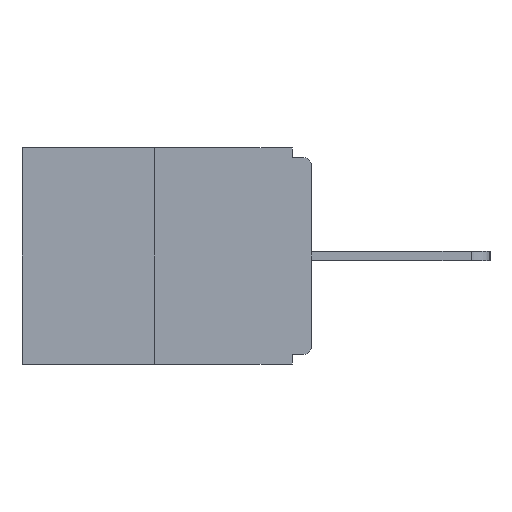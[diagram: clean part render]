
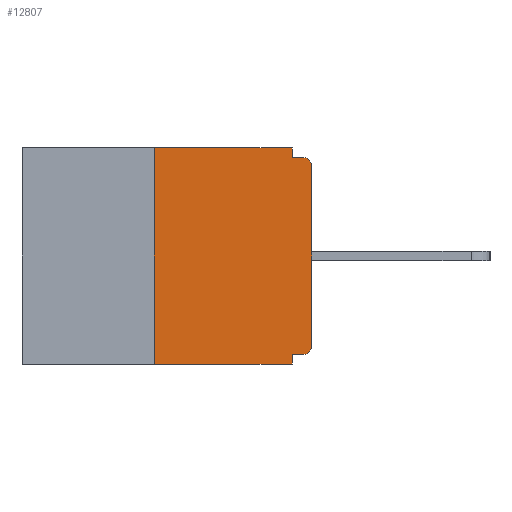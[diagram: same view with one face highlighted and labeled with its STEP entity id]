
A CAD part, left-side view. The second image highlights one B-rep face of the part: STEP entity #12807.
In plain terms, the highlighted planar face has unit normal (-1, 0, 0).
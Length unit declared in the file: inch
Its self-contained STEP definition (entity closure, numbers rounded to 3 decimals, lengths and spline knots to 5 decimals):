
#68 = CARTESIAN_POINT ( 'NONE',  ( 0., 0.031, 0. ) ) ;
#231 = AXIS2_PLACEMENT_3D ( 'NONE', #5222, #12648, #6312 ) ;
#589 = VERTEX_POINT ( 'NONE', #12794 ) ;
#752 = VECTOR ( 'NONE', #6473, 39.37008 ) ;
#1267 = VERTEX_POINT ( 'NONE', #9443 ) ;
#1361 = EDGE_CURVE ( 'NONE', #7565, #2502, #13836, .T. ) ;
#1569 = CARTESIAN_POINT ( 'NONE',  ( 0., 0., -0.313 ) ) ;
#1834 = ORIENTED_EDGE ( 'NONE', *, *, #4089, .F. ) ;
#2036 = VERTEX_POINT ( 'NONE', #1569 ) ;
#2199 = ORIENTED_EDGE ( 'NONE', *, *, #1361, .T. ) ;
#2500 = CARTESIAN_POINT ( 'NONE',  ( 0., 0.015, -0.015 ) ) ;
#2502 = VERTEX_POINT ( 'NONE', #7137 ) ;
#2579 = CARTESIAN_POINT ( 'NONE',  ( 0., 0., -0.03 ) ) ;
#2752 = CARTESIAN_POINT ( 'NONE',  ( 0., 0.46, 0. ) ) ;
#2889 = DIRECTION ( 'NONE',  ( 0., 0., -1. ) ) ;
#2912 = DIRECTION ( 'NONE',  ( 0., -1., 0. ) ) ;
#3065 = EDGE_LOOP ( 'NONE', ( #12920, #1834, #2199, #13422, #8104, #5618, #12589, #13583, #11748, #3576 ) ) ;
#3076 = CARTESIAN_POINT ( 'NONE',  ( 0., 0.46, -0.343 ) ) ;
#3139 = VECTOR ( 'NONE', #6002, 39.37008 ) ;
#3576 = ORIENTED_EDGE ( 'NONE', *, *, #10837, .F. ) ;
#3677 = CARTESIAN_POINT ( 'NONE',  ( 0., 0.015, -0.03 ) ) ;
#3810 = CARTESIAN_POINT ( 'NONE',  ( 0., 0.46, 0. ) ) ;
#3862 = DIRECTION ( 'NONE',  ( 0., 0., -1. ) ) ;
#4089 = EDGE_CURVE ( 'NONE', #7565, #5576, #6040, .T. ) ;
#4292 = CARTESIAN_POINT ( 'NONE',  ( 0., 0.031, -0.343 ) ) ;
#4603 = VECTOR ( 'NONE', #12014, 39.37008 ) ;
#4623 = CARTESIAN_POINT ( 'NONE',  ( 0., 0.25, 0. ) ) ;
#4667 = AXIS2_PLACEMENT_3D ( 'NONE', #3677, #11118, #4792 ) ;
#4774 = VECTOR ( 'NONE', #5253, 39.37008 ) ;
#4792 = DIRECTION ( 'NONE',  ( 0., 0., -1. ) ) ;
#5140 = CARTESIAN_POINT ( 'NONE',  ( 0., 0.031, 0. ) ) ;
#5148 = CARTESIAN_POINT ( 'NONE',  ( 0., 0., 0. ) ) ;
#5222 = CARTESIAN_POINT ( 'NONE',  ( 0., 0.015, -0.313 ) ) ;
#5253 = DIRECTION ( 'NONE',  ( 0., 1., 0. ) ) ;
#5353 = CARTESIAN_POINT ( 'NONE',  ( 0., 0.015, -0.328 ) ) ;
#5357 = VECTOR ( 'NONE', #2912, 39.37008 ) ;
#5427 = VECTOR ( 'NONE', #11240, 39.37008 ) ;
#5576 = VERTEX_POINT ( 'NONE', #10037 ) ;
#5618 = ORIENTED_EDGE ( 'NONE', *, *, #7032, .T. ) ;
#5628 = VERTEX_POINT ( 'NONE', #2579 ) ;
#6002 = DIRECTION ( 'NONE',  ( 0., 0., 1. ) ) ;
#6040 = LINE ( 'NONE', #4623, #3139 ) ;
#6144 = VERTEX_POINT ( 'NONE', #68 ) ;
#6312 = DIRECTION ( 'NONE',  ( 0., 0., -1. ) ) ;
#6473 = DIRECTION ( 'NONE',  ( 0., 0., -1. ) ) ;
#6479 = EDGE_CURVE ( 'NONE', #2036, #5628, #6979, .T. ) ;
#6979 = LINE ( 'NONE', #5148, #10102 ) ;
#7032 = EDGE_CURVE ( 'NONE', #9244, #2036, #8125, .T. ) ;
#7137 = CARTESIAN_POINT ( 'NONE',  ( 0., 0.031, -0.343 ) ) ;
#7565 = VERTEX_POINT ( 'NONE', #12486 ) ;
#7654 = EDGE_CURVE ( 'NONE', #9244, #1267, #7935, .T. ) ;
#7754 = EDGE_CURVE ( 'NONE', #1267, #2502, #9425, .T. ) ;
#7930 = EDGE_CURVE ( 'NONE', #589, #13283, #9907, .T. ) ;
#7935 = LINE ( 'NONE', #10523, #4774 ) ;
#8104 = ORIENTED_EDGE ( 'NONE', *, *, #7654, .F. ) ;
#8113 = EDGE_CURVE ( 'NONE', #5576, #6144, #11045, .T. ) ;
#8125 = CIRCLE ( 'NONE', #231, 0.015 ) ;
#9028 = FACE_OUTER_BOUND ( 'NONE', #3065, .T. ) ;
#9068 = LINE ( 'NONE', #5140, #11209 ) ;
#9169 = PLANE ( 'NONE',  #12614 ) ;
#9244 = VERTEX_POINT ( 'NONE', #5353 ) ;
#9425 = LINE ( 'NONE', #4292, #752 ) ;
#9443 = CARTESIAN_POINT ( 'NONE',  ( 0., 0.031, -0.328 ) ) ;
#9907 = LINE ( 'NONE', #10930, #4603 ) ;
#10037 = CARTESIAN_POINT ( 'NONE',  ( 0., 0.25, 0. ) ) ;
#10102 = VECTOR ( 'NONE', #13632, 39.37008 ) ;
#10226 = DIRECTION ( 'NONE',  ( 1., 0., 0. ) ) ;
#10523 = CARTESIAN_POINT ( 'NONE',  ( 0., 0., -0.328 ) ) ;
#10837 = EDGE_CURVE ( 'NONE', #6144, #589, #9068, .T. ) ;
#10930 = CARTESIAN_POINT ( 'NONE',  ( 0., 0., -0.015 ) ) ;
#11045 = LINE ( 'NONE', #3810, #5427 ) ;
#11118 = DIRECTION ( 'NONE',  ( -1., 0., 0. ) ) ;
#11209 = VECTOR ( 'NONE', #2889, 39.37008 ) ;
#11240 = DIRECTION ( 'NONE',  ( 0., -1., 0. ) ) ;
#11262 = EDGE_CURVE ( 'NONE', #5628, #13283, #11893, .T. ) ;
#11748 = ORIENTED_EDGE ( 'NONE', *, *, #7930, .F. ) ;
#11893 = CIRCLE ( 'NONE', #4667, 0.015 ) ;
#12014 = DIRECTION ( 'NONE',  ( 0., -1., 0. ) ) ;
#12486 = CARTESIAN_POINT ( 'NONE',  ( 0., 0.25, -0.343 ) ) ;
#12589 = ORIENTED_EDGE ( 'NONE', *, *, #6479, .T. ) ;
#12614 = AXIS2_PLACEMENT_3D ( 'NONE', #2752, #10226, #3862 ) ;
#12648 = DIRECTION ( 'NONE',  ( -1., 0., 0. ) ) ;
#12794 = CARTESIAN_POINT ( 'NONE',  ( 0., 0.031, -0.015 ) ) ;
#12807 = ADVANCED_FACE ( 'NONE', ( #9028 ), #9169, .F. ) ;
#12920 = ORIENTED_EDGE ( 'NONE', *, *, #8113, .F. ) ;
#13283 = VERTEX_POINT ( 'NONE', #2500 ) ;
#13422 = ORIENTED_EDGE ( 'NONE', *, *, #7754, .F. ) ;
#13583 = ORIENTED_EDGE ( 'NONE', *, *, #11262, .T. ) ;
#13632 = DIRECTION ( 'NONE',  ( 0., 0., 1. ) ) ;
#13836 = LINE ( 'NONE', #3076, #5357 ) ;
